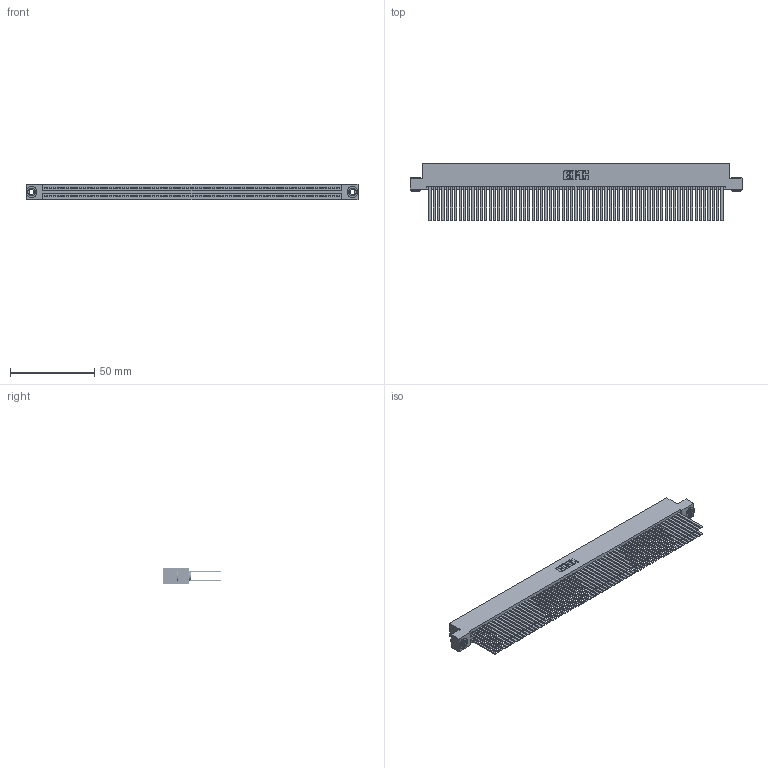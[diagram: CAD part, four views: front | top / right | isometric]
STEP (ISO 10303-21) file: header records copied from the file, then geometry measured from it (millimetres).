
FILE_DESCRIPTION (( 'STEP AP203' ), '1' );
FILE_NAME ('345-138-544-203.STEP', '2018-10-20T19:30:48', ( '' ), ( '' ), 'SwSTEP 2.0', 'SolidWorks 2016', '' );
FILE_SCHEMA (( 'CONFIG_CONTROL_DESIGN' ));
Length unit declared in the file: inch
Products named in the file (4): 345-250-002_345-250-002-102; 345-292-001_345-293-144; 345-138-544-203; 345 Part_Flush Mounting Lugs - 0.156 Dia-TH
Assembly tree (141 placements, depth 2):
  345-138-544-203
    345 Part_Flush Mounting Lugs - 0.156 Dia-TH
    345-292-001_345-293-144  x138
    345-250-002_345-250-002-102  x2
Bounding box: 196.47 x 33.96 x 9.4 mm (x, y, z)
Volume: 21289.7 mm3; surface area: 37867.5 mm2
Topology: 141 solids, 141 shells, 6236 faces, 18495 edges, 12142 vertices
Faces by surface type: plane 4092, cylinder 2136, cone 8
Entity records: 50970 total; most frequent: CARTESIAN_POINT 8491, ORIENTED_EDGE 8418, DIRECTION 7483, EDGE_CURVE 4209, LINE 3781, VECTOR 3781, VERTEX_POINT 2802, AXIS2_PLACEMENT_3D 1851
